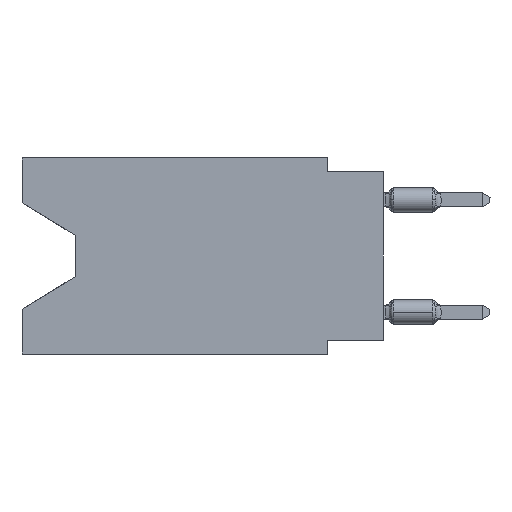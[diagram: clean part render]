
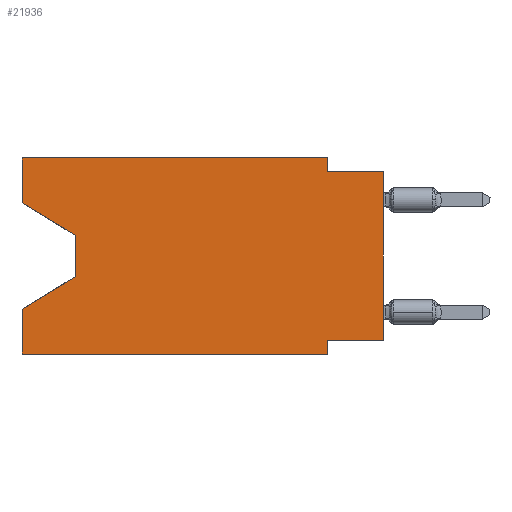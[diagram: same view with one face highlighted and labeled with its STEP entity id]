
A CAD part, left-side view. The second image highlights one B-rep face of the part: STEP entity #21936.
In plain terms, the highlighted planar face has unit normal (-1, 0, 0).
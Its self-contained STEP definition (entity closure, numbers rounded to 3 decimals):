
#113 = CARTESIAN_POINT ( 'NONE',  ( 0., 16.383, 0. ) ) ;
#254 = VECTOR ( 'NONE', #22269, 1000. ) ;
#283 = EDGE_CURVE ( 'NONE', #15674, #18623, #12164, .T. ) ;
#419 = CARTESIAN_POINT ( 'NONE',  ( 0., 16.383, -2.038 ) ) ;
#1314 = LINE ( 'NONE', #23702, #16019 ) ;
#1912 = CARTESIAN_POINT ( 'NONE',  ( 0., 16.383, 0. ) ) ;
#2275 = EDGE_CURVE ( 'NONE', #8697, #15674, #20585, .T. ) ;
#2412 = DIRECTION ( 'NONE',  ( 1., 0., 0. ) ) ;
#2443 = VERTEX_POINT ( 'NONE', #7887 ) ;
#2533 = LINE ( 'NONE', #10536, #23656 ) ;
#2643 = EDGE_CURVE ( 'NONE', #19101, #20814, #20553, .T. ) ;
#2928 = VECTOR ( 'NONE', #17175, 1000. ) ;
#2929 = CARTESIAN_POINT ( 'NONE',  ( 0., 16.383, -8.89 ) ) ;
#3420 = AXIS2_PLACEMENT_3D ( 'NONE', #21381, #2412, #9922 ) ;
#3599 = EDGE_CURVE ( 'NONE', #20814, #8697, #7677, .T. ) ;
#3722 = DIRECTION ( 'NONE',  ( 0., 0.855, -0.519 ) ) ;
#4295 = ORIENTED_EDGE ( 'NONE', *, *, #20621, .T. ) ;
#4603 = VECTOR ( 'NONE', #15733, 1000. ) ;
#5039 = EDGE_CURVE ( 'NONE', #7931, #21426, #18285, .T. ) ;
#5144 = ORIENTED_EDGE ( 'NONE', *, *, #283, .F. ) ;
#5568 = ORIENTED_EDGE ( 'NONE', *, *, #18834, .F. ) ;
#6026 = VECTOR ( 'NONE', #16985, 1000. ) ;
#6218 = EDGE_CURVE ( 'NONE', #2443, #7931, #16860, .T. ) ;
#6485 = LINE ( 'NONE', #9470, #23181 ) ;
#6611 = CARTESIAN_POINT ( 'NONE',  ( 0., 0., -0.635 ) ) ;
#6783 = ORIENTED_EDGE ( 'NONE', *, *, #19372, .T. ) ;
#6902 = VECTOR ( 'NONE', #3722, 1000. ) ;
#7012 = LINE ( 'NONE', #24000, #19299 ) ;
#7176 = CARTESIAN_POINT ( 'NONE',  ( 0., 2.54, 0. ) ) ;
#7243 = CARTESIAN_POINT ( 'NONE',  ( 0., 13.97, -3.505 ) ) ;
#7284 = DIRECTION ( 'NONE',  ( 0., 0., -1. ) ) ;
#7296 = CARTESIAN_POINT ( 'NONE',  ( 0., 13.97, -5.385 ) ) ;
#7677 = LINE ( 'NONE', #1912, #2928 ) ;
#7887 = CARTESIAN_POINT ( 'NONE',  ( 0., 13.97, -3.505 ) ) ;
#7931 = VERTEX_POINT ( 'NONE', #18860 ) ;
#8697 = VERTEX_POINT ( 'NONE', #7176 ) ;
#8771 = VECTOR ( 'NONE', #7284, 1000. ) ;
#9461 = ORIENTED_EDGE ( 'NONE', *, *, #20076, .F. ) ;
#9470 = CARTESIAN_POINT ( 'NONE',  ( 0., 16.383, -8.89 ) ) ;
#9714 = VERTEX_POINT ( 'NONE', #2929 ) ;
#9918 = CARTESIAN_POINT ( 'NONE',  ( 0., 0., -0.635 ) ) ;
#9922 = DIRECTION ( 'NONE',  ( 0., 0., -1. ) ) ;
#10050 = PLANE ( 'NONE',  #3420 ) ;
#10390 = ORIENTED_EDGE ( 'NONE', *, *, #2643, .F. ) ;
#10496 = CARTESIAN_POINT ( 'NONE',  ( 0., 2.54, -8.89 ) ) ;
#10536 = CARTESIAN_POINT ( 'NONE',  ( 0., 2.54, -8.89 ) ) ;
#10933 = CARTESIAN_POINT ( 'NONE',  ( 0., 16.383, -2.038 ) ) ;
#11008 = CARTESIAN_POINT ( 'NONE',  ( 0., 2.54, -0.635 ) ) ;
#11891 = CARTESIAN_POINT ( 'NONE',  ( 0., 2.54, -8.255 ) ) ;
#11915 = DIRECTION ( 'NONE',  ( 0., -1., 0. ) ) ;
#12103 = ORIENTED_EDGE ( 'NONE', *, *, #3599, .F. ) ;
#12164 = LINE ( 'NONE', #6611, #4603 ) ;
#12397 = ORIENTED_EDGE ( 'NONE', *, *, #22109, .F. ) ;
#12514 = CARTESIAN_POINT ( 'NONE',  ( 0., 16.383, 0. ) ) ;
#12720 = LINE ( 'NONE', #16893, #13696 ) ;
#12795 = ORIENTED_EDGE ( 'NONE', *, *, #6218, .T. ) ;
#12972 = ORIENTED_EDGE ( 'NONE', *, *, #2275, .F. ) ;
#13377 = EDGE_CURVE ( 'NONE', #15755, #18623, #12720, .T. ) ;
#13696 = VECTOR ( 'NONE', #18753, 1000. ) ;
#13850 = DIRECTION ( 'NONE',  ( 0., 0., -1. ) ) ;
#14665 = ORIENTED_EDGE ( 'NONE', *, *, #5039, .T. ) ;
#15039 = CARTESIAN_POINT ( 'NONE',  ( 0., 16.383, -6.852 ) ) ;
#15578 = EDGE_LOOP ( 'NONE', ( #4295, #12795, #14665, #12397, #6783, #5568, #9461, #22872, #5144, #12972, #12103, #10390 ) ) ;
#15587 = VECTOR ( 'NONE', #18689, 1000. ) ;
#15674 = VERTEX_POINT ( 'NONE', #11008 ) ;
#15733 = DIRECTION ( 'NONE',  ( 0., -1., 0. ) ) ;
#15755 = VERTEX_POINT ( 'NONE', #23326 ) ;
#16019 = VECTOR ( 'NONE', #16211, 1000. ) ;
#16211 = DIRECTION ( 'NONE',  ( 0., 0., 1. ) ) ;
#16349 = VERTEX_POINT ( 'NONE', #10496 ) ;
#16860 = LINE ( 'NONE', #7243, #254 ) ;
#16893 = CARTESIAN_POINT ( 'NONE',  ( 0., 0., 0. ) ) ;
#16985 = DIRECTION ( 'NONE',  ( 0., 0., 1. ) ) ;
#17175 = DIRECTION ( 'NONE',  ( 0., -1., 0. ) ) ;
#18285 = LINE ( 'NONE', #7296, #6902 ) ;
#18623 = VERTEX_POINT ( 'NONE', #9918 ) ;
#18677 = VERTEX_POINT ( 'NONE', #11891 ) ;
#18689 = DIRECTION ( 'NONE',  ( 0., -0.855, -0.519 ) ) ;
#18753 = DIRECTION ( 'NONE',  ( 0., 0., 1. ) ) ;
#18834 = EDGE_CURVE ( 'NONE', #18677, #16349, #2533, .T. ) ;
#18860 = CARTESIAN_POINT ( 'NONE',  ( 0., 13.97, -5.385 ) ) ;
#19060 = FACE_OUTER_BOUND ( 'NONE', #15578, .T. ) ;
#19101 = VERTEX_POINT ( 'NONE', #419 ) ;
#19299 = VECTOR ( 'NONE', #22036, 1000. ) ;
#19372 = EDGE_CURVE ( 'NONE', #9714, #16349, #6485, .T. ) ;
#20076 = EDGE_CURVE ( 'NONE', #15755, #18677, #7012, .T. ) ;
#20472 = CARTESIAN_POINT ( 'NONE',  ( 0., 2.54, 0. ) ) ;
#20553 = LINE ( 'NONE', #113, #6026 ) ;
#20585 = LINE ( 'NONE', #20472, #8771 ) ;
#20621 = EDGE_CURVE ( 'NONE', #19101, #2443, #24089, .T. ) ;
#20814 = VERTEX_POINT ( 'NONE', #12514 ) ;
#21381 = CARTESIAN_POINT ( 'NONE',  ( 0., 16.383, 0. ) ) ;
#21426 = VERTEX_POINT ( 'NONE', #15039 ) ;
#21936 = ADVANCED_FACE ( 'NONE', ( #19060 ), #10050, .F. ) ;
#22036 = DIRECTION ( 'NONE',  ( 0., 1., 0. ) ) ;
#22109 = EDGE_CURVE ( 'NONE', #9714, #21426, #1314, .T. ) ;
#22269 = DIRECTION ( 'NONE',  ( 0., 0., -1. ) ) ;
#22872 = ORIENTED_EDGE ( 'NONE', *, *, #13377, .T. ) ;
#23181 = VECTOR ( 'NONE', #11915, 1000. ) ;
#23326 = CARTESIAN_POINT ( 'NONE',  ( 0., 0., -8.255 ) ) ;
#23656 = VECTOR ( 'NONE', #13850, 1000. ) ;
#23702 = CARTESIAN_POINT ( 'NONE',  ( 0., 16.383, 0. ) ) ;
#24000 = CARTESIAN_POINT ( 'NONE',  ( 0., 0., -8.255 ) ) ;
#24089 = LINE ( 'NONE', #10933, #15587 ) ;
